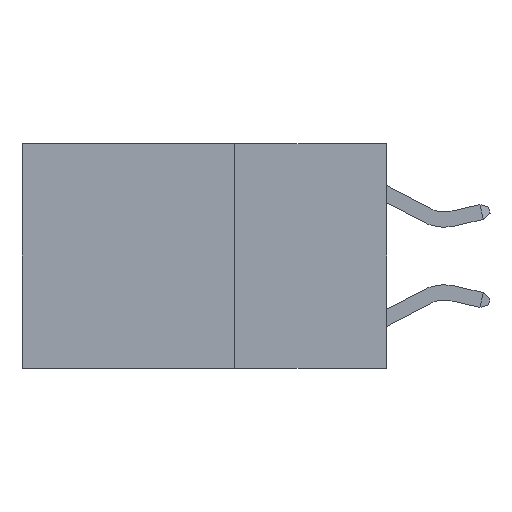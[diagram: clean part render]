
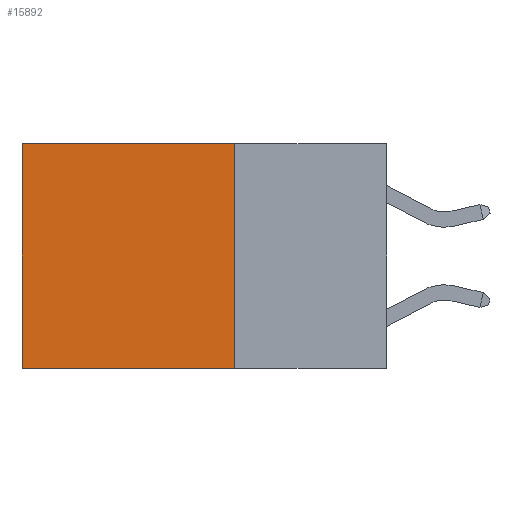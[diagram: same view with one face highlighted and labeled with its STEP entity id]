
A CAD part, left-side view. The second image highlights one B-rep face of the part: STEP entity #15892.
In plain terms, the highlighted planar face has unit normal (-1, 0, 0).
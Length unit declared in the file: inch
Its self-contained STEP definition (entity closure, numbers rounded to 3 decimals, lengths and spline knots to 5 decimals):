
#804 = FACE_OUTER_BOUND ( 'NONE', #11030, .T. ) ;
#811 = DIRECTION ( 'NONE',  ( 1., 0., 0. ) ) ;
#1107 = ORIENTED_EDGE ( 'NONE', *, *, #13868, .T. ) ;
#1981 = VERTEX_POINT ( 'NONE', #2577 ) ;
#2091 = CARTESIAN_POINT ( 'NONE',  ( 0.2625, 0.6, -0.37 ) ) ;
#2278 = CARTESIAN_POINT ( 'NONE',  ( 0.2625, 0.25, -0.37 ) ) ;
#2577 = CARTESIAN_POINT ( 'NONE',  ( 0.2625, 0.6, 0. ) ) ;
#3482 = EDGE_CURVE ( 'NONE', #11610, #7896, #8232, .T. ) ;
#3510 = VECTOR ( 'NONE', #5331, 39.37008 ) ;
#3985 = VECTOR ( 'NONE', #14683, 39.37008 ) ;
#4256 = VECTOR ( 'NONE', #12654, 39.37008 ) ;
#5331 = DIRECTION ( 'NONE',  ( 0., 0., -1. ) ) ;
#7043 = CARTESIAN_POINT ( 'NONE',  ( 0.2625, 0.6, 0. ) ) ;
#7101 = CARTESIAN_POINT ( 'NONE',  ( 0.2625, 0.25, 0. ) ) ;
#7896 = VERTEX_POINT ( 'NONE', #9256 ) ;
#8117 = CARTESIAN_POINT ( 'NONE',  ( 0.2625, 0.25, 0. ) ) ;
#8232 = LINE ( 'NONE', #12199, #3510 ) ;
#9049 = ORIENTED_EDGE ( 'NONE', *, *, #16185, .T. ) ;
#9256 = CARTESIAN_POINT ( 'NONE',  ( 0.2625, 0.25, -0.37 ) ) ;
#9626 = LINE ( 'NONE', #7043, #4256 ) ;
#9911 = LINE ( 'NONE', #7101, #10793 ) ;
#10339 = ORIENTED_EDGE ( 'NONE', *, *, #3482, .F. ) ;
#10793 = VECTOR ( 'NONE', #12467, 39.37008 ) ;
#10801 = AXIS2_PLACEMENT_3D ( 'NONE', #17175, #811, #17120 ) ;
#11030 = EDGE_LOOP ( 'NONE', ( #9049, #13141, #10339, #1107 ) ) ;
#11610 = VERTEX_POINT ( 'NONE', #8117 ) ;
#12199 = CARTESIAN_POINT ( 'NONE',  ( 0.2625, 0.25, 0. ) ) ;
#12467 = DIRECTION ( 'NONE',  ( 0., 1., 0. ) ) ;
#12654 = DIRECTION ( 'NONE',  ( 0., 0., -1. ) ) ;
#12827 = LINE ( 'NONE', #2278, #3985 ) ;
#13141 = ORIENTED_EDGE ( 'NONE', *, *, #17313, .F. ) ;
#13868 = EDGE_CURVE ( 'NONE', #11610, #1981, #9911, .T. ) ;
#14668 = PLANE ( 'NONE',  #10801 ) ;
#14683 = DIRECTION ( 'NONE',  ( 0., 1., 0. ) ) ;
#15314 = VERTEX_POINT ( 'NONE', #2091 ) ;
#15892 = ADVANCED_FACE ( 'NONE', ( #804 ), #14668, .F. ) ;
#16185 = EDGE_CURVE ( 'NONE', #1981, #15314, #9626, .T. ) ;
#17120 = DIRECTION ( 'NONE',  ( 0., 0., -1. ) ) ;
#17175 = CARTESIAN_POINT ( 'NONE',  ( 0.2625, 0.25, 0. ) ) ;
#17313 = EDGE_CURVE ( 'NONE', #7896, #15314, #12827, .T. ) ;
